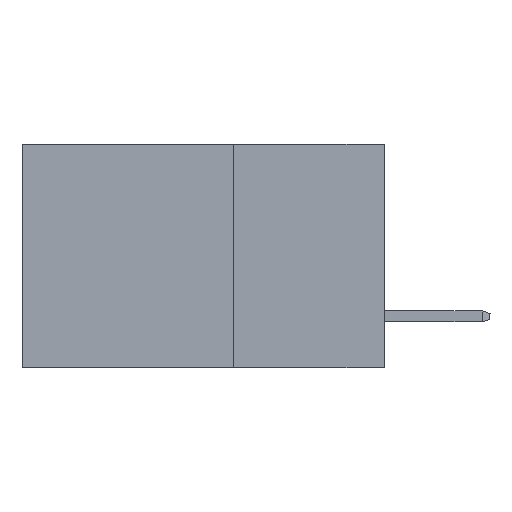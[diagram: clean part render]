
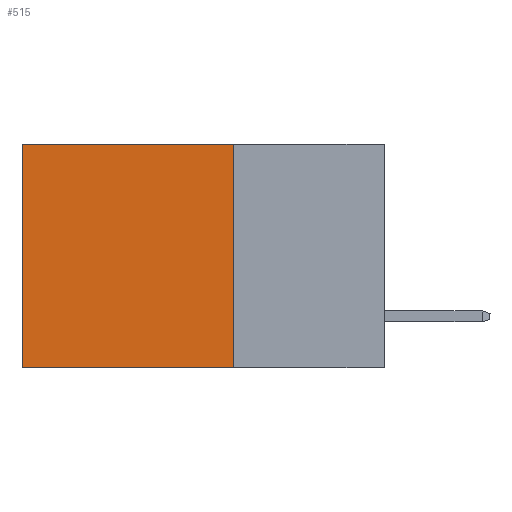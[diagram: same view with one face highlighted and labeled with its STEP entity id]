
A CAD part, left-side view. The second image highlights one B-rep face of the part: STEP entity #515.
In plain terms, the highlighted planar face has unit normal (-1, 0, 0).
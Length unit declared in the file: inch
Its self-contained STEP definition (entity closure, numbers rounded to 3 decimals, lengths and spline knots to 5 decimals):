
#515 = ADVANCED_FACE ( 'NONE', ( #12454 ), #19658, .F. ) ;
#678 = CARTESIAN_POINT ( 'NONE',  ( 0.2615, 0.25, 0. ) ) ;
#1302 = EDGE_LOOP ( 'NONE', ( #2157, #2625, #5079, #9811 ) ) ;
#1806 = CARTESIAN_POINT ( 'NONE',  ( 0.2615, 0.25, -0.37 ) ) ;
#1808 = DIRECTION ( 'NONE',  ( 0., 0., -1. ) ) ;
#2157 = ORIENTED_EDGE ( 'NONE', *, *, #3941, .T. ) ;
#2568 = LINE ( 'NONE', #678, #23088 ) ;
#2625 = ORIENTED_EDGE ( 'NONE', *, *, #5178, .F. ) ;
#2741 = CARTESIAN_POINT ( 'NONE',  ( 0.2615, 0.25, -0.37 ) ) ;
#3164 = VERTEX_POINT ( 'NONE', #17418 ) ;
#3529 = LINE ( 'NONE', #17917, #18351 ) ;
#3831 = VERTEX_POINT ( 'NONE', #4943 ) ;
#3941 = EDGE_CURVE ( 'NONE', #3831, #21459, #3529, .T. ) ;
#4532 = VECTOR ( 'NONE', #1808, 39.37008 ) ;
#4943 = CARTESIAN_POINT ( 'NONE',  ( 0.2615, 0.6, 0. ) ) ;
#5079 = ORIENTED_EDGE ( 'NONE', *, *, #15003, .F. ) ;
#5178 = EDGE_CURVE ( 'NONE', #3164, #21459, #10072, .T. ) ;
#5407 = CARTESIAN_POINT ( 'NONE',  ( 0.2615, 0.25, 0. ) ) ;
#6267 = DIRECTION ( 'NONE',  ( 0., 1., 0. ) ) ;
#7232 = DIRECTION ( 'NONE',  ( 0., 0., -1. ) ) ;
#7760 = DIRECTION ( 'NONE',  ( 0., 0., -1. ) ) ;
#9020 = DIRECTION ( 'NONE',  ( 1., 0., 0. ) ) ;
#9811 = ORIENTED_EDGE ( 'NONE', *, *, #18055, .T. ) ;
#10072 = LINE ( 'NONE', #2741, #22831 ) ;
#10748 = VERTEX_POINT ( 'NONE', #5407 ) ;
#12454 = FACE_OUTER_BOUND ( 'NONE', #1302, .T. ) ;
#12683 = CARTESIAN_POINT ( 'NONE',  ( 0.2615, 0.25, -0.37 ) ) ;
#13183 = DIRECTION ( 'NONE',  ( 0., 1., 0. ) ) ;
#14572 = LINE ( 'NONE', #12683, #4532 ) ;
#15003 = EDGE_CURVE ( 'NONE', #10748, #3164, #14572, .T. ) ;
#16980 = AXIS2_PLACEMENT_3D ( 'NONE', #1806, #9020, #7232 ) ;
#17418 = CARTESIAN_POINT ( 'NONE',  ( 0.2615, 0.25, -0.37 ) ) ;
#17917 = CARTESIAN_POINT ( 'NONE',  ( 0.2615, 0.6, -0.37 ) ) ;
#18055 = EDGE_CURVE ( 'NONE', #10748, #3831, #2568, .T. ) ;
#18216 = CARTESIAN_POINT ( 'NONE',  ( 0.2615, 0.6, -0.37 ) ) ;
#18351 = VECTOR ( 'NONE', #7760, 39.37008 ) ;
#19658 = PLANE ( 'NONE',  #16980 ) ;
#21459 = VERTEX_POINT ( 'NONE', #18216 ) ;
#22831 = VECTOR ( 'NONE', #6267, 39.37008 ) ;
#23088 = VECTOR ( 'NONE', #13183, 39.37008 ) ;
